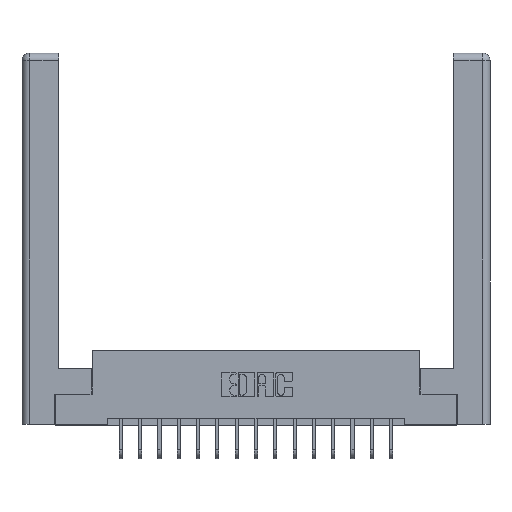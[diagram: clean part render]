
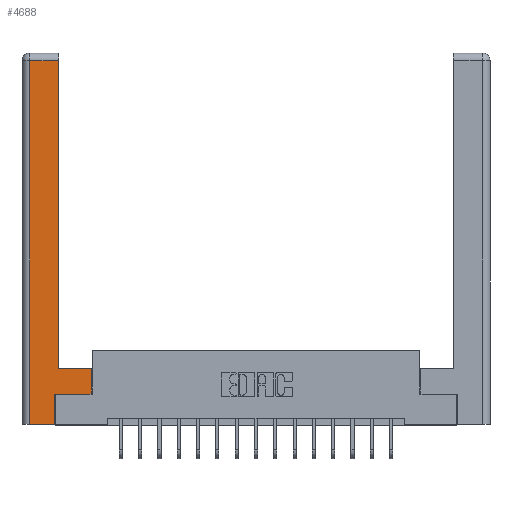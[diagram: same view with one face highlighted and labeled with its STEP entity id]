
A CAD part, top view. The second image highlights one B-rep face of the part: STEP entity #4688.
In plain terms, the highlighted planar face has unit normal (0, 0, 1).
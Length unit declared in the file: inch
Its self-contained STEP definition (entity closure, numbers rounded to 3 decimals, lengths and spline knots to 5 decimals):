
#70 = EDGE_CURVE ( 'NONE', #3500, #4406, #10216, .T. ) ;
#157 = CARTESIAN_POINT ( 'NONE',  ( 0.565, 0.45, 0. ) ) ;
#254 = EDGE_CURVE ( 'NONE', #4406, #1846, #6210, .T. ) ;
#978 = VECTOR ( 'NONE', #10395, 39.37008 ) ;
#1027 = CARTESIAN_POINT ( 'NONE',  ( 0.265, 0.245, 0. ) ) ;
#1046 = VECTOR ( 'NONE', #13660, 39.37008 ) ;
#1132 = CARTESIAN_POINT ( 'NONE',  ( 0.265, 0.245, 0. ) ) ;
#1846 = VERTEX_POINT ( 'NONE', #6803 ) ;
#2105 = VERTEX_POINT ( 'NONE', #1132 ) ;
#2562 = CARTESIAN_POINT ( 'NONE',  ( 0.265, 0., 0. ) ) ;
#3002 = CARTESIAN_POINT ( 'NONE',  ( 0.0615, 0., 0. ) ) ;
#3314 = DIRECTION ( 'NONE',  ( -1., 0., 0. ) ) ;
#3500 = VERTEX_POINT ( 'NONE', #5392 ) ;
#3583 = DIRECTION ( 'NONE',  ( 0., 1., 0. ) ) ;
#3915 = DIRECTION ( 'NONE',  ( -1., 0., 0. ) ) ;
#4052 = ORIENTED_EDGE ( 'NONE', *, *, #70, .T. ) ;
#4115 = LINE ( 'NONE', #5236, #11045 ) ;
#4120 = VECTOR ( 'NONE', #10995, 39.37008 ) ;
#4128 = LINE ( 'NONE', #14954, #16089 ) ;
#4344 = AXIS2_PLACEMENT_3D ( 'NONE', #9852, #11381, #3314 ) ;
#4406 = VERTEX_POINT ( 'NONE', #7412 ) ;
#4688 = ADVANCED_FACE ( 'NONE', ( #6467 ), #16694, .F. ) ;
#5236 = CARTESIAN_POINT ( 'NONE',  ( 0.565, 0.245, 0. ) ) ;
#5392 = CARTESIAN_POINT ( 'NONE',  ( 0.295, 0.45, 0. ) ) ;
#5832 = EDGE_CURVE ( 'NONE', #1846, #8923, #4128, .T. ) ;
#6210 = LINE ( 'NONE', #13154, #978 ) ;
#6458 = DIRECTION ( 'NONE',  ( 1., 0., 0. ) ) ;
#6467 = FACE_OUTER_BOUND ( 'NONE', #12451, .T. ) ;
#6803 = CARTESIAN_POINT ( 'NONE',  ( 0.0615, 2.94, 0. ) ) ;
#7412 = CARTESIAN_POINT ( 'NONE',  ( 0.295, 2.94, 0. ) ) ;
#7635 = ORIENTED_EDGE ( 'NONE', *, *, #5832, .T. ) ;
#7902 = LINE ( 'NONE', #11980, #14202 ) ;
#7922 = VECTOR ( 'NONE', #8009, 39.37008 ) ;
#8009 = DIRECTION ( 'NONE',  ( 1., 0., 0. ) ) ;
#8144 = CARTESIAN_POINT ( 'NONE',  ( 0.265, 0., 0. ) ) ;
#8585 = LINE ( 'NONE', #15121, #1046 ) ;
#8923 = VERTEX_POINT ( 'NONE', #3002 ) ;
#9852 = CARTESIAN_POINT ( 'NONE',  ( 0., 0., 0. ) ) ;
#10216 = LINE ( 'NONE', #16493, #4120 ) ;
#10395 = DIRECTION ( 'NONE',  ( -1., 0., 0. ) ) ;
#10478 = EDGE_CURVE ( 'NONE', #16799, #15402, #8585, .T. ) ;
#10995 = DIRECTION ( 'NONE',  ( 0., 1., 0. ) ) ;
#11045 = VECTOR ( 'NONE', #6458, 39.37008 ) ;
#11133 = CARTESIAN_POINT ( 'NONE',  ( 0.565, 0.245, 0. ) ) ;
#11381 = DIRECTION ( 'NONE',  ( 0., 0., -1. ) ) ;
#11519 = LINE ( 'NONE', #2562, #7922 ) ;
#11967 = ORIENTED_EDGE ( 'NONE', *, *, #12221, .T. ) ;
#11980 = CARTESIAN_POINT ( 'NONE',  ( 0.295, 0.45, 0. ) ) ;
#12153 = DIRECTION ( 'NONE',  ( 0., -1., 0. ) ) ;
#12156 = EDGE_CURVE ( 'NONE', #8923, #15944, #11519, .T. ) ;
#12221 = EDGE_CURVE ( 'NONE', #15402, #3500, #7902, .T. ) ;
#12451 = EDGE_LOOP ( 'NONE', ( #4052, #14128, #7635, #15044, #15989, #15260, #16091, #11967 ) ) ;
#12900 = VECTOR ( 'NONE', #3583, 39.37008 ) ;
#13154 = CARTESIAN_POINT ( 'NONE',  ( 0.0615, 2.94, 0. ) ) ;
#13660 = DIRECTION ( 'NONE',  ( 0., 1., 0. ) ) ;
#13939 = LINE ( 'NONE', #1027, #12900 ) ;
#14128 = ORIENTED_EDGE ( 'NONE', *, *, #254, .T. ) ;
#14181 = EDGE_CURVE ( 'NONE', #15944, #2105, #13939, .T. ) ;
#14202 = VECTOR ( 'NONE', #3915, 39.37008 ) ;
#14954 = CARTESIAN_POINT ( 'NONE',  ( 0.0615, 0., 0. ) ) ;
#15044 = ORIENTED_EDGE ( 'NONE', *, *, #12156, .T. ) ;
#15121 = CARTESIAN_POINT ( 'NONE',  ( 0.565, 0.45, 0. ) ) ;
#15260 = ORIENTED_EDGE ( 'NONE', *, *, #17188, .T. ) ;
#15402 = VERTEX_POINT ( 'NONE', #157 ) ;
#15944 = VERTEX_POINT ( 'NONE', #8144 ) ;
#15989 = ORIENTED_EDGE ( 'NONE', *, *, #14181, .T. ) ;
#16089 = VECTOR ( 'NONE', #12153, 39.37008 ) ;
#16091 = ORIENTED_EDGE ( 'NONE', *, *, #10478, .T. ) ;
#16493 = CARTESIAN_POINT ( 'NONE',  ( 0.295, 3., 0. ) ) ;
#16694 = PLANE ( 'NONE',  #4344 ) ;
#16799 = VERTEX_POINT ( 'NONE', #11133 ) ;
#17188 = EDGE_CURVE ( 'NONE', #2105, #16799, #4115, .T. ) ;
